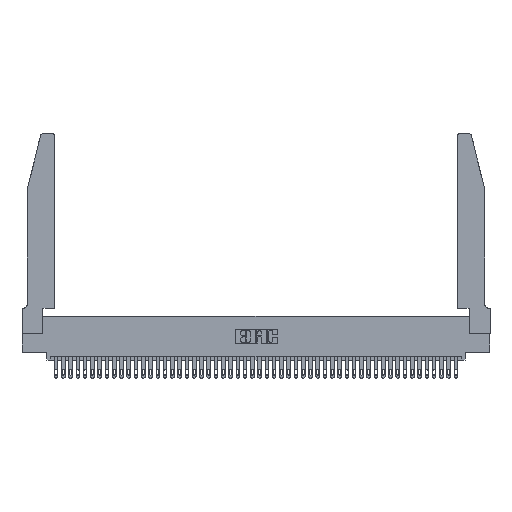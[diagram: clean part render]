
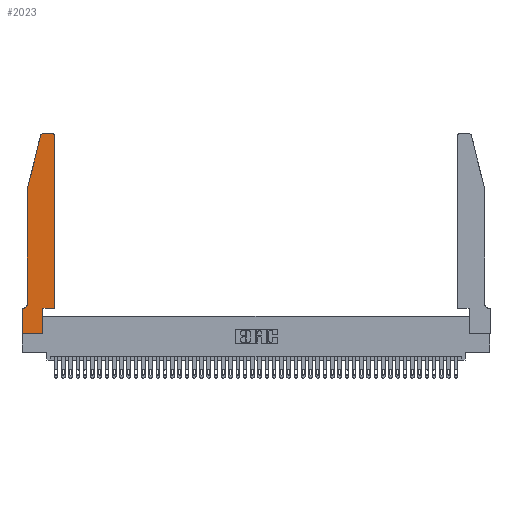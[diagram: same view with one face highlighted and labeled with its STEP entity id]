
A CAD part, top view. The second image highlights one B-rep face of the part: STEP entity #2023.
In plain terms, the highlighted planar face has unit normal (0, 0, 1).
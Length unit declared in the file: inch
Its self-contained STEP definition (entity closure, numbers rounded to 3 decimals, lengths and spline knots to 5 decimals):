
#2023 = ADVANCED_FACE ( 'NONE', ( #3000 ), #5630, .T. ) ;
#2987 = EDGE_CURVE ( 'NONE', #18750, #36025, #14314, .T. ) ;
#3000 = FACE_OUTER_BOUND ( 'NONE', #39787, .T. ) ;
#3270 = EDGE_CURVE ( 'NONE', #24219, #37356, #8566, .T. ) ;
#3998 = DIRECTION ( 'NONE',  ( 1., 0., 0. ) ) ;
#4629 = ORIENTED_EDGE ( 'NONE', *, *, #31077, .T. ) ;
#4877 = VECTOR ( 'NONE', #6708, 39.37008 ) ;
#5101 = CARTESIAN_POINT ( 'NONE',  ( 0.284, 2.72, 0.37 ) ) ;
#5487 = VECTOR ( 'NONE', #7878, 39.37008 ) ;
#5630 = PLANE ( 'NONE',  #33098 ) ;
#5893 = EDGE_CURVE ( 'NONE', #41326, #11753, #45135, .T. ) ;
#6063 = CARTESIAN_POINT ( 'NONE',  ( 0., 0., 0.37 ) ) ;
#6708 = DIRECTION ( 'NONE',  ( 0., 1., 0. ) ) ;
#6805 = VERTEX_POINT ( 'NONE', #26863 ) ;
#7878 = DIRECTION ( 'NONE',  ( 1., 0., 0. ) ) ;
#7935 = CARTESIAN_POINT ( 'NONE',  ( 0.0055, 0.42, 0.37 ) ) ;
#8566 = LINE ( 'NONE', #35768, #38011 ) ;
#8727 = EDGE_CURVE ( 'NONE', #11753, #24219, #44844, .T. ) ;
#10071 = CARTESIAN_POINT ( 'NONE',  ( 0.2865, 0.35, 0.37 ) ) ;
#10945 = ORIENTED_EDGE ( 'NONE', *, *, #15272, .T. ) ;
#11753 = VERTEX_POINT ( 'NONE', #39957 ) ;
#12239 = DIRECTION ( 'NONE',  ( 0., 0., -1. ) ) ;
#12406 = DIRECTION ( 'NONE',  ( 0., 0., 1. ) ) ;
#12621 = CARTESIAN_POINT ( 'NONE',  ( 0.2865, 0.35, 0.37 ) ) ;
#12754 = ORIENTED_EDGE ( 'NONE', *, *, #22066, .T. ) ;
#12797 = DIRECTION ( 'NONE',  ( 0., 0., 1. ) ) ;
#12813 = ORIENTED_EDGE ( 'NONE', *, *, #18270, .T. ) ;
#12823 = CARTESIAN_POINT ( 'NONE',  ( 0.0755, 2., 0.37 ) ) ;
#14314 = CIRCLE ( 'NONE', #28892, 0.03 ) ;
#14364 = ORIENTED_EDGE ( 'NONE', *, *, #33592, .T. ) ;
#14899 = DIRECTION ( 'NONE',  ( 0., -1., 0. ) ) ;
#14913 = VERTEX_POINT ( 'NONE', #23016 ) ;
#15272 = EDGE_CURVE ( 'NONE', #6805, #41326, #27625, .T. ) ;
#16060 = ORIENTED_EDGE ( 'NONE', *, *, #46192, .T. ) ;
#16585 = CARTESIAN_POINT ( 'NONE',  ( 0.0055, 0.35, 0.37 ) ) ;
#16776 = VECTOR ( 'NONE', #46703, 39.37008 ) ;
#16847 = AXIS2_PLACEMENT_3D ( 'NONE', #33986, #12797, #30234 ) ;
#18270 = EDGE_CURVE ( 'NONE', #39504, #14913, #41442, .T. ) ;
#18750 = VERTEX_POINT ( 'NONE', #30170 ) ;
#19489 = EDGE_CURVE ( 'NONE', #21755, #34031, #44222, .T. ) ;
#21755 = VERTEX_POINT ( 'NONE', #38180 ) ;
#22066 = EDGE_CURVE ( 'NONE', #36025, #41782, #32163, .T. ) ;
#22167 = DIRECTION ( 'NONE',  ( 1., 0., 0. ) ) ;
#22837 = DIRECTION ( 'NONE',  ( -0.239, -0.971, 0. ) ) ;
#23016 = CARTESIAN_POINT ( 'NONE',  ( 0.4205, 2.75, 0.37 ) ) ;
#23203 = CARTESIAN_POINT ( 'NONE',  ( 0.4505, 0.35, 0.37 ) ) ;
#24219 = VERTEX_POINT ( 'NONE', #12621 ) ;
#25111 = ORIENTED_EDGE ( 'NONE', *, *, #3270, .T. ) ;
#25365 = AXIS2_PLACEMENT_3D ( 'NONE', #7935, #12239, #33285 ) ;
#26277 = EDGE_CURVE ( 'NONE', #41782, #21755, #32229, .T. ) ;
#26719 = VECTOR ( 'NONE', #42158, 39.37008 ) ;
#26863 = CARTESIAN_POINT ( 'NONE',  ( 0., 0.35, 0.37 ) ) ;
#27587 = LINE ( 'NONE', #35326, #4877 ) ;
#27625 = LINE ( 'NONE', #42078, #29316 ) ;
#28892 = AXIS2_PLACEMENT_3D ( 'NONE', #5101, #12406, #41307 ) ;
#29316 = VECTOR ( 'NONE', #45257, 39.37008 ) ;
#30143 = CARTESIAN_POINT ( 'NONE',  ( 0.0755, 2., 0.37 ) ) ;
#30170 = CARTESIAN_POINT ( 'NONE',  ( 0.284, 2.75, 0.37 ) ) ;
#30234 = DIRECTION ( 'NONE',  ( 1., 0., 0. ) ) ;
#30478 = VECTOR ( 'NONE', #22837, 39.37008 ) ;
#31077 = EDGE_CURVE ( 'NONE', #14913, #18750, #34649, .T. ) ;
#31269 = CARTESIAN_POINT ( 'NONE',  ( 0.4505, 2.72, 0.37 ) ) ;
#31301 = CARTESIAN_POINT ( 'NONE',  ( 0.2605, 2.75, 0.37 ) ) ;
#31386 = ORIENTED_EDGE ( 'NONE', *, *, #8727, .T. ) ;
#32163 = LINE ( 'NONE', #30143, #30478 ) ;
#32229 = LINE ( 'NONE', #36546, #33319 ) ;
#32387 = DIRECTION ( 'NONE',  ( 0., 0., 1. ) ) ;
#33098 = AXIS2_PLACEMENT_3D ( 'NONE', #43095, #32387, #3998 ) ;
#33285 = DIRECTION ( 'NONE',  ( -1., 0., 0. ) ) ;
#33319 = VECTOR ( 'NONE', #14899, 39.37008 ) ;
#33592 = EDGE_CURVE ( 'NONE', #34031, #6805, #33756, .T. ) ;
#33756 = LINE ( 'NONE', #43040, #16776 ) ;
#33986 = CARTESIAN_POINT ( 'NONE',  ( 0.4205, 2.72, 0.37 ) ) ;
#34031 = VERTEX_POINT ( 'NONE', #16585 ) ;
#34649 = LINE ( 'NONE', #31301, #26719 ) ;
#34757 = DIRECTION ( 'NONE',  ( 0., 1., 0. ) ) ;
#35326 = CARTESIAN_POINT ( 'NONE',  ( 0.4505, 0.35, 0.37 ) ) ;
#35768 = CARTESIAN_POINT ( 'NONE',  ( 0.4505, 0.35, 0.37 ) ) ;
#36025 = VERTEX_POINT ( 'NONE', #37986 ) ;
#36445 = ORIENTED_EDGE ( 'NONE', *, *, #19489, .T. ) ;
#36546 = CARTESIAN_POINT ( 'NONE',  ( 0.0755, 2., 0.37 ) ) ;
#37231 = CARTESIAN_POINT ( 'NONE',  ( 0., 0., 0.37 ) ) ;
#37356 = VERTEX_POINT ( 'NONE', #23203 ) ;
#37986 = CARTESIAN_POINT ( 'NONE',  ( 0.25487, 2.72718, 0.37 ) ) ;
#38011 = VECTOR ( 'NONE', #22167, 39.37008 ) ;
#38180 = CARTESIAN_POINT ( 'NONE',  ( 0.0755, 0.42, 0.37 ) ) ;
#39504 = VERTEX_POINT ( 'NONE', #31269 ) ;
#39787 = EDGE_LOOP ( 'NONE', ( #4629, #42648, #12754, #40346, #36445, #14364, #10945, #43712, #31386, #25111, #16060, #12813 ) ) ;
#39957 = CARTESIAN_POINT ( 'NONE',  ( 0.2865, 0., 0.37 ) ) ;
#40346 = ORIENTED_EDGE ( 'NONE', *, *, #26277, .T. ) ;
#41307 = DIRECTION ( 'NONE',  ( 1., 0., 0. ) ) ;
#41326 = VERTEX_POINT ( 'NONE', #6063 ) ;
#41422 = VECTOR ( 'NONE', #34757, 39.37008 ) ;
#41442 = CIRCLE ( 'NONE', #16847, 0.03 ) ;
#41782 = VERTEX_POINT ( 'NONE', #12823 ) ;
#42078 = CARTESIAN_POINT ( 'NONE',  ( 0., 0., 0.37 ) ) ;
#42158 = DIRECTION ( 'NONE',  ( -1., 0., 0. ) ) ;
#42648 = ORIENTED_EDGE ( 'NONE', *, *, #2987, .T. ) ;
#43040 = CARTESIAN_POINT ( 'NONE',  ( 0.0755, 0.35, 0.37 ) ) ;
#43095 = CARTESIAN_POINT ( 'NONE',  ( 0., 0.35, 0.37 ) ) ;
#43712 = ORIENTED_EDGE ( 'NONE', *, *, #5893, .T. ) ;
#44222 = CIRCLE ( 'NONE', #25365, 0.07 ) ;
#44844 = LINE ( 'NONE', #10071, #41422 ) ;
#45135 = LINE ( 'NONE', #37231, #5487 ) ;
#45257 = DIRECTION ( 'NONE',  ( 0., -1., 0. ) ) ;
#46192 = EDGE_CURVE ( 'NONE', #37356, #39504, #27587, .T. ) ;
#46703 = DIRECTION ( 'NONE',  ( -1., 0., 0. ) ) ;
